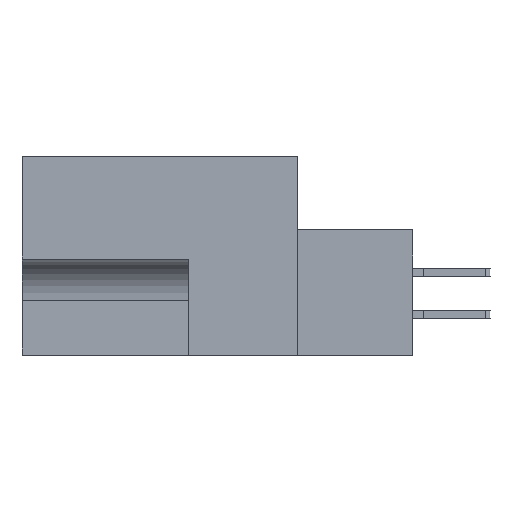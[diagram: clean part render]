
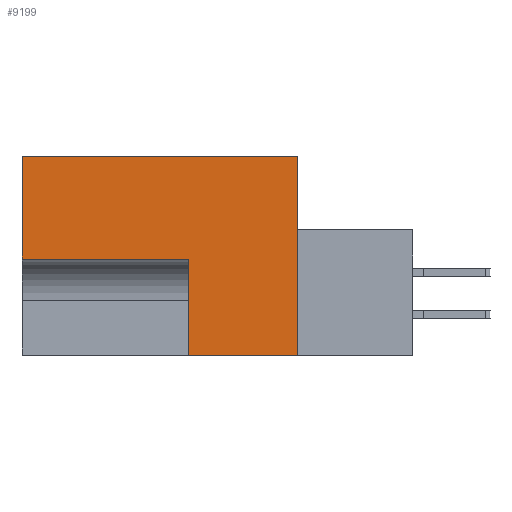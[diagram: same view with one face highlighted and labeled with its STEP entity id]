
A CAD part, left-side view. The second image highlights one B-rep face of the part: STEP entity #9199.
In plain terms, the highlighted planar face has unit normal (-1, 0, 0).
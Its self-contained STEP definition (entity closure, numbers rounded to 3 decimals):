
#2368 = VERTEX_POINT ( 'NONE', #28294 ) ;
#2448 = VERTEX_POINT ( 'NONE', #24470 ) ;
#2816 = VECTOR ( 'NONE', #9054, 1000. ) ;
#4849 = EDGE_CURVE ( 'NONE', #34179, #26098, #44711, .T. ) ;
#5563 = CARTESIAN_POINT ( 'NONE',  ( 0., 0., 0. ) ) ;
#5912 = EDGE_CURVE ( 'NONE', #18647, #34179, #30404, .T. ) ;
#6619 = VECTOR ( 'NONE', #16724, 1000. ) ;
#7482 = CARTESIAN_POINT ( 'NONE',  ( 0., 0., 0. ) ) ;
#8571 = EDGE_CURVE ( 'NONE', #41744, #18647, #37644, .T. ) ;
#9054 = DIRECTION ( 'NONE',  ( 0., 1., 0. ) ) ;
#9199 = ADVANCED_FACE ( 'NONE', ( #36372 ), #31473, .F. ) ;
#11532 = ORIENTED_EDGE ( 'NONE', *, *, #4849, .F. ) ;
#12080 = CARTESIAN_POINT ( 'NONE',  ( 0., 20.955, -15.088 ) ) ;
#12386 = DIRECTION ( 'NONE',  ( 1., 0., 0. ) ) ;
#15879 = DIRECTION ( 'NONE',  ( 0., 0., -1. ) ) ;
#16724 = DIRECTION ( 'NONE',  ( 0., 0., 1. ) ) ;
#17196 = ORIENTED_EDGE ( 'NONE', *, *, #8571, .F. ) ;
#18269 = ORIENTED_EDGE ( 'NONE', *, *, #42198, .F. ) ;
#18647 = VERTEX_POINT ( 'NONE', #50815 ) ;
#19371 = ORIENTED_EDGE ( 'NONE', *, *, #31420, .F. ) ;
#19870 = EDGE_LOOP ( 'NONE', ( #17196, #18269, #41552, #19371, #11532, #25275 ) ) ;
#22267 = AXIS2_PLACEMENT_3D ( 'NONE', #7482, #12386, #15879 ) ;
#24470 = CARTESIAN_POINT ( 'NONE',  ( 0., 20.955, 0. ) ) ;
#25275 = ORIENTED_EDGE ( 'NONE', *, *, #5912, .F. ) ;
#26098 = VERTEX_POINT ( 'NONE', #40520 ) ;
#28146 = CARTESIAN_POINT ( 'NONE',  ( 0., -8.814, -15.088 ) ) ;
#28294 = CARTESIAN_POINT ( 'NONE',  ( 0., 0., 0. ) ) ;
#28910 = VECTOR ( 'NONE', #32172, 1000. ) ;
#29589 = VECTOR ( 'NONE', #39547, 1000. ) ;
#30404 = LINE ( 'NONE', #37022, #6619 ) ;
#31420 = EDGE_CURVE ( 'NONE', #26098, #2448, #50138, .T. ) ;
#31473 = PLANE ( 'NONE',  #22267 ) ;
#32172 = DIRECTION ( 'NONE',  ( 0., 1., 0. ) ) ;
#34125 = CARTESIAN_POINT ( 'NONE',  ( 0., 0., -15.088 ) ) ;
#34179 = VERTEX_POINT ( 'NONE', #39948 ) ;
#35324 = CARTESIAN_POINT ( 'NONE',  ( 0., 11.506, 0. ) ) ;
#35425 = LINE ( 'NONE', #5563, #41067 ) ;
#35574 = EDGE_CURVE ( 'NONE', #2448, #2368, #48301, .T. ) ;
#36196 = DIRECTION ( 'NONE',  ( 0., 0., 1. ) ) ;
#36372 = FACE_OUTER_BOUND ( 'NONE', #19870, .T. ) ;
#36852 = CARTESIAN_POINT ( 'NONE',  ( 0., 8.255, -7.772 ) ) ;
#37022 = CARTESIAN_POINT ( 'NONE',  ( 0., 8.255, -15.088 ) ) ;
#37644 = LINE ( 'NONE', #28146, #28910 ) ;
#39547 = DIRECTION ( 'NONE',  ( 0., -1., 0. ) ) ;
#39552 = VECTOR ( 'NONE', #36196, 1000. ) ;
#39948 = CARTESIAN_POINT ( 'NONE',  ( 0., 8.255, -7.772 ) ) ;
#40520 = CARTESIAN_POINT ( 'NONE',  ( 0., 20.955, -7.772 ) ) ;
#41067 = VECTOR ( 'NONE', #49413, 1000. ) ;
#41552 = ORIENTED_EDGE ( 'NONE', *, *, #35574, .F. ) ;
#41744 = VERTEX_POINT ( 'NONE', #34125 ) ;
#42198 = EDGE_CURVE ( 'NONE', #2368, #41744, #35425, .T. ) ;
#44711 = LINE ( 'NONE', #36852, #2816 ) ;
#48301 = LINE ( 'NONE', #35324, #29589 ) ;
#49413 = DIRECTION ( 'NONE',  ( 0., 0., -1. ) ) ;
#50138 = LINE ( 'NONE', #12080, #39552 ) ;
#50815 = CARTESIAN_POINT ( 'NONE',  ( 0., 8.255, -15.088 ) ) ;
